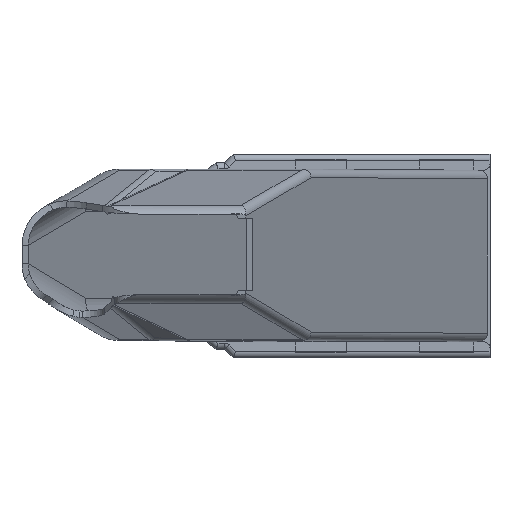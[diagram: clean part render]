
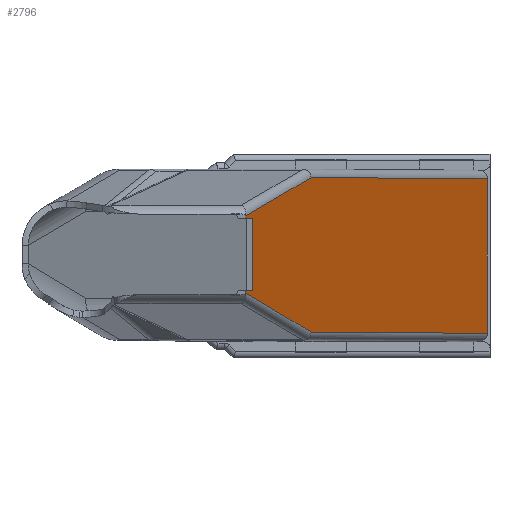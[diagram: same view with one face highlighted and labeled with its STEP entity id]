
A CAD part, top view. The second image highlights one B-rep face of the part: STEP entity #2796.
In plain terms, the highlighted planar face has unit normal (0.966, 0, 0.259).
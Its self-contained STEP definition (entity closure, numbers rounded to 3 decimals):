
#248=PLANE('',#3076);
#1012=ORIENTED_EDGE('',*,*,#1525,.T.);
#1013=ORIENTED_EDGE('',*,*,#1439,.T.);
#1014=ORIENTED_EDGE('',*,*,#1435,.F.);
#1015=ORIENTED_EDGE('',*,*,#1433,.F.);
#1016=ORIENTED_EDGE('',*,*,#1430,.F.);
#1017=ORIENTED_EDGE('',*,*,#1427,.F.);
#1018=ORIENTED_EDGE('',*,*,#1423,.F.);
#1019=ORIENTED_EDGE('',*,*,#1422,.T.);
#1020=ORIENTED_EDGE('',*,*,#1524,.T.);
#1021=ORIENTED_EDGE('',*,*,#1526,.T.);
#1422=EDGE_CURVE('',#1756,#1757,#1976,.F.);
#1423=EDGE_CURVE('',#1756,#1758,#1977,.T.);
#1427=EDGE_CURVE('',#1758,#1760,#1981,.F.);
#1430=EDGE_CURVE('',#1760,#1762,#1984,.F.);
#1433=EDGE_CURVE('',#1762,#1763,#1987,.F.);
#1435=EDGE_CURVE('',#1763,#1764,#1988,.T.);
#1439=EDGE_CURVE('',#1768,#1764,#1990,.T.);
#1524=EDGE_CURVE('',#1757,#1813,#2048,.F.);
#1525=EDGE_CURVE('',#1814,#1768,#2049,.T.);
#1526=EDGE_CURVE('',#1813,#1814,#2050,.F.);
#1756=VERTEX_POINT('',#4734);
#1757=VERTEX_POINT('',#4736);
#1758=VERTEX_POINT('',#4740);
#1760=VERTEX_POINT('',#4745);
#1762=VERTEX_POINT('',#4751);
#1763=VERTEX_POINT('',#4756);
#1764=VERTEX_POINT('',#4761);
#1768=VERTEX_POINT('',#4772);
#1813=VERTEX_POINT('',#4947);
#1814=VERTEX_POINT('',#4951);
#1976=LINE('',#4737,#2214);
#1977=LINE('',#4739,#2215);
#1981=LINE('',#4747,#2219);
#1984=LINE('',#4753,#2222);
#1987=LINE('',#4758,#2225);
#1988=LINE('',#4762,#2226);
#1990=LINE('',#4771,#2228);
#2048=LINE('',#4948,#2286);
#2049=LINE('',#4950,#2287);
#2050=LINE('',#4952,#2288);
#2214=VECTOR('',#3600,1000.);
#2215=VECTOR('',#3603,1000.);
#2219=VECTOR('',#3609,1000.);
#2222=VECTOR('',#3614,1000.);
#2225=VECTOR('',#3619,1000.);
#2226=VECTOR('',#3624,1000.);
#2228=VECTOR('',#3634,1000.);
#2286=VECTOR('',#3806,1000.);
#2287=VECTOR('',#3809,1000.);
#2288=VECTOR('',#3810,1000.);
#2435=EDGE_LOOP('',(#1012,#1013,#1014,#1015,#1016,#1017,#1018,#1019,#1020,
#1021));
#2588=FACE_BOUND('',#2435,.T.);
#2796=ADVANCED_FACE('',(#2588),#248,.T.);
#3076=AXIS2_PLACEMENT_3D('',#4949,#3807,#3808);
#3600=DIRECTION('',(-0.256,0.152,0.955));
#3603=DIRECTION('',(0.,1.,0.));
#3609=DIRECTION('',(-0.259,0.,0.966));
#3614=DIRECTION('',(0.,-1.,0.));
#3619=DIRECTION('',(0.259,-0.005,-0.966));
#3624=DIRECTION('',(0.,1.,0.));
#3634=DIRECTION('',(-0.256,-0.152,0.955));
#3806=DIRECTION('',(-0.259,0.,0.966));
#3807=DIRECTION('',(0.966,0.,0.259));
#3808=DIRECTION('',(0.259,0.,-0.966));
#3809=DIRECTION('',(-0.259,0.,0.966));
#3810=DIRECTION('',(0.,-1.,0.));
#4734=CARTESIAN_POINT('',(129.127,-4.528,-1.748));
#4736=CARTESIAN_POINT('',(136.844,-9.1,-30.55));
#4737=CARTESIAN_POINT('',(156.376,-20.671,-103.443));
#4739=CARTESIAN_POINT('',(129.127,-16.397,-1.748));
#4740=CARTESIAN_POINT('',(129.127,-4.25,-1.748));
#4745=CARTESIAN_POINT('',(129.903,-4.25,-4.646));
#4747=CARTESIAN_POINT('',(129.903,-4.25,-4.646));
#4751=CARTESIAN_POINT('',(129.903,4.25,-4.646));
#4753=CARTESIAN_POINT('',(129.903,0.,-4.646));
#4756=CARTESIAN_POINT('',(129.127,4.266,-1.748));
#4758=CARTESIAN_POINT('',(129.903,4.25,-4.646));
#4761=CARTESIAN_POINT('',(129.127,4.528,-1.748));
#4762=CARTESIAN_POINT('',(129.127,-16.397,-1.748));
#4771=CARTESIAN_POINT('',(129.164,4.55,-1.889));
#4772=CARTESIAN_POINT('',(136.844,9.1,-30.55));
#4947=CARTESIAN_POINT('',(157.597,-9.1,-108.));
#4948=CARTESIAN_POINT('',(157.597,-9.1,-108.));
#4949=CARTESIAN_POINT('',(157.597,10.1,-108.));
#4950=CARTESIAN_POINT('',(157.597,9.1,-108.));
#4951=CARTESIAN_POINT('',(157.597,9.1,-108.));
#4952=CARTESIAN_POINT('',(157.597,10.1,-108.));
